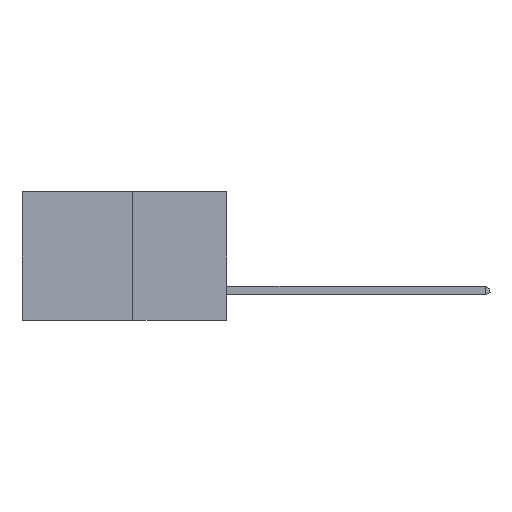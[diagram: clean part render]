
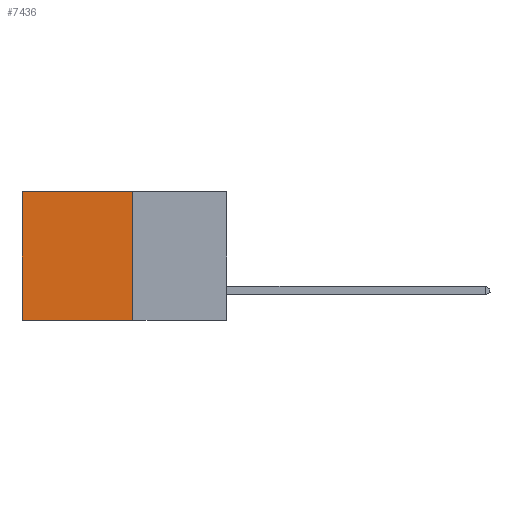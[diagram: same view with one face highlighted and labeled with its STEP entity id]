
A CAD part, left-side view. The second image highlights one B-rep face of the part: STEP entity #7436.
In plain terms, the highlighted planar face has unit normal (-1, 0, 0).
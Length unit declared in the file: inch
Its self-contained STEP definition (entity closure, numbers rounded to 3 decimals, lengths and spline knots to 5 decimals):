
#271 = EDGE_CURVE ( 'NONE', #8258, #6007, #10605, .T. ) ;
#411 = CARTESIAN_POINT ( 'NONE',  ( 0.277, 0.27, -0.37 ) ) ;
#443 = LINE ( 'NONE', #6673, #3076 ) ;
#540 = DIRECTION ( 'NONE',  ( 0., 0., -1. ) ) ;
#898 = VERTEX_POINT ( 'NONE', #5472 ) ;
#1130 = EDGE_CURVE ( 'NONE', #898, #8258, #7346, .T. ) ;
#1195 = CARTESIAN_POINT ( 'NONE',  ( 0.277, 0.27, 0. ) ) ;
#1419 = DIRECTION ( 'NONE',  ( 0., 1., 0. ) ) ;
#1670 = VECTOR ( 'NONE', #2035, 39.37008 ) ;
#2035 = DIRECTION ( 'NONE',  ( 0., 0., -1. ) ) ;
#2467 = CARTESIAN_POINT ( 'NONE',  ( 0.277, 0.59, -0.37 ) ) ;
#2914 = EDGE_CURVE ( 'NONE', #898, #10185, #8069, .T. ) ;
#3076 = VECTOR ( 'NONE', #540, 39.37008 ) ;
#4324 = CARTESIAN_POINT ( 'NONE',  ( 0.277, 0.27, -0.37 ) ) ;
#4637 = CARTESIAN_POINT ( 'NONE',  ( 0.277, 0.59, 0. ) ) ;
#5472 = CARTESIAN_POINT ( 'NONE',  ( 0.277, 0.27, 0. ) ) ;
#5709 = PLANE ( 'NONE',  #6889 ) ;
#6007 = VERTEX_POINT ( 'NONE', #2467 ) ;
#6555 = DIRECTION ( 'NONE',  ( 0., 1., 0. ) ) ;
#6673 = CARTESIAN_POINT ( 'NONE',  ( 0.277, 0.59, -0.37 ) ) ;
#6677 = DIRECTION ( 'NONE',  ( 0., 0., -1. ) ) ;
#6889 = AXIS2_PLACEMENT_3D ( 'NONE', #9518, #12278, #6677 ) ;
#6910 = ORIENTED_EDGE ( 'NONE', *, *, #1130, .F. ) ;
#7346 = LINE ( 'NONE', #12055, #1670 ) ;
#7436 = ADVANCED_FACE ( 'NONE', ( #9273 ), #5709, .F. ) ;
#8069 = LINE ( 'NONE', #1195, #12667 ) ;
#8258 = VERTEX_POINT ( 'NONE', #411 ) ;
#9147 = ORIENTED_EDGE ( 'NONE', *, *, #9211, .T. ) ;
#9199 = EDGE_LOOP ( 'NONE', ( #9147, #11607, #6910, #11882 ) ) ;
#9211 = EDGE_CURVE ( 'NONE', #10185, #6007, #443, .T. ) ;
#9273 = FACE_OUTER_BOUND ( 'NONE', #9199, .T. ) ;
#9518 = CARTESIAN_POINT ( 'NONE',  ( 0.277, 0.27, -0.37 ) ) ;
#10185 = VERTEX_POINT ( 'NONE', #4637 ) ;
#10312 = VECTOR ( 'NONE', #6555, 39.37008 ) ;
#10605 = LINE ( 'NONE', #4324, #10312 ) ;
#11607 = ORIENTED_EDGE ( 'NONE', *, *, #271, .F. ) ;
#11882 = ORIENTED_EDGE ( 'NONE', *, *, #2914, .T. ) ;
#12055 = CARTESIAN_POINT ( 'NONE',  ( 0.277, 0.27, -0.37 ) ) ;
#12278 = DIRECTION ( 'NONE',  ( 1., 0., 0. ) ) ;
#12667 = VECTOR ( 'NONE', #1419, 39.37008 ) ;
